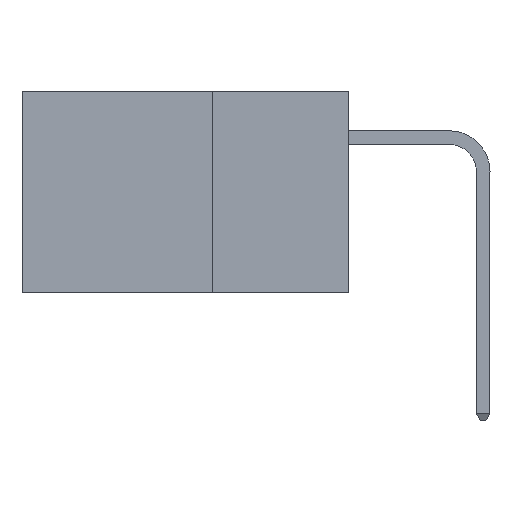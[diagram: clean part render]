
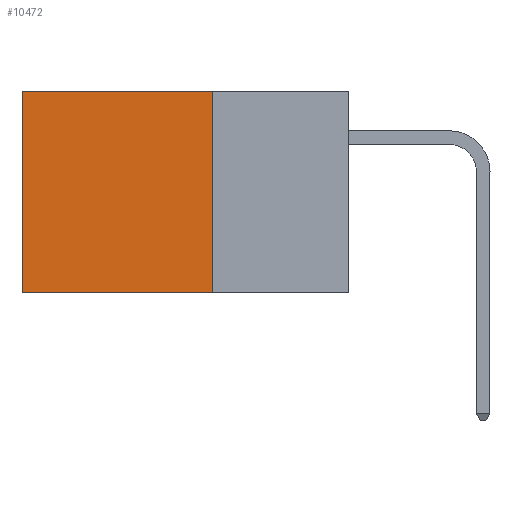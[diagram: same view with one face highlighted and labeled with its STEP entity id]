
A CAD part, left-side view. The second image highlights one B-rep face of the part: STEP entity #10472.
In plain terms, the highlighted planar face has unit normal (-1, 0, 0).
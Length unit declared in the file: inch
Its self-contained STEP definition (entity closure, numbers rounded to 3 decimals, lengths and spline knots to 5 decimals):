
#2878 = FACE_OUTER_BOUND ( 'NONE', #32744, .T. ) ;
#4463 = DIRECTION ( 'NONE',  ( 0., 1., 0. ) ) ;
#4523 = EDGE_CURVE ( 'NONE', #27661, #35113, #31811, .T. ) ;
#4820 = CARTESIAN_POINT ( 'NONE',  ( 0.2875, 0.25, 0. ) ) ;
#6457 = ORIENTED_EDGE ( 'NONE', *, *, #4523, .T. ) ;
#7738 = DIRECTION ( 'NONE',  ( 0., 0., -1. ) ) ;
#8747 = ORIENTED_EDGE ( 'NONE', *, *, #16575, .T. ) ;
#10472 = ADVANCED_FACE ( 'NONE', ( #2878 ), #18908, .F. ) ;
#11465 = ORIENTED_EDGE ( 'NONE', *, *, #11912, .F. ) ;
#11912 = EDGE_CURVE ( 'NONE', #19590, #35367, #18721, .T. ) ;
#13011 = VECTOR ( 'NONE', #4463, 39.37008 ) ;
#14904 = EDGE_CURVE ( 'NONE', #35367, #35113, #27253, .T. ) ;
#15763 = CARTESIAN_POINT ( 'NONE',  ( 0.2875, 0.25, 0. ) ) ;
#16575 = EDGE_CURVE ( 'NONE', #19590, #27661, #20424, .T. ) ;
#17871 = CARTESIAN_POINT ( 'NONE',  ( 0.2875, 0.6, 0. ) ) ;
#18721 = LINE ( 'NONE', #30470, #25244 ) ;
#18908 = PLANE ( 'NONE',  #25400 ) ;
#19590 = VERTEX_POINT ( 'NONE', #19698 ) ;
#19698 = CARTESIAN_POINT ( 'NONE',  ( 0.2875, 0.25, 0. ) ) ;
#20142 = ORIENTED_EDGE ( 'NONE', *, *, #14904, .F. ) ;
#20424 = LINE ( 'NONE', #15763, #13011 ) ;
#20791 = DIRECTION ( 'NONE',  ( 0., 0., -1. ) ) ;
#21387 = CARTESIAN_POINT ( 'NONE',  ( 0.2875, 0.6, -0.37 ) ) ;
#22335 = CARTESIAN_POINT ( 'NONE',  ( 0.2875, 0.25, -0.37 ) ) ;
#24490 = VECTOR ( 'NONE', #20791, 39.37008 ) ;
#24526 = DIRECTION ( 'NONE',  ( 1., 0., 0. ) ) ;
#24630 = VECTOR ( 'NONE', #33227, 39.37008 ) ;
#25244 = VECTOR ( 'NONE', #35969, 39.37008 ) ;
#25400 = AXIS2_PLACEMENT_3D ( 'NONE', #4820, #24526, #7738 ) ;
#27253 = LINE ( 'NONE', #27717, #24630 ) ;
#27661 = VERTEX_POINT ( 'NONE', #29627 ) ;
#27717 = CARTESIAN_POINT ( 'NONE',  ( 0.2875, 0.25, -0.37 ) ) ;
#29627 = CARTESIAN_POINT ( 'NONE',  ( 0.2875, 0.6, 0. ) ) ;
#30470 = CARTESIAN_POINT ( 'NONE',  ( 0.2875, 0.25, 0. ) ) ;
#31811 = LINE ( 'NONE', #17871, #24490 ) ;
#32744 = EDGE_LOOP ( 'NONE', ( #6457, #20142, #11465, #8747 ) ) ;
#33227 = DIRECTION ( 'NONE',  ( 0., 1., 0. ) ) ;
#35113 = VERTEX_POINT ( 'NONE', #21387 ) ;
#35367 = VERTEX_POINT ( 'NONE', #22335 ) ;
#35969 = DIRECTION ( 'NONE',  ( 0., 0., -1. ) ) ;
